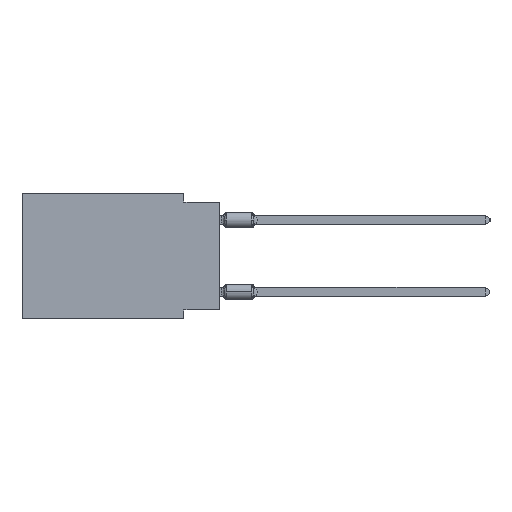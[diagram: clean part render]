
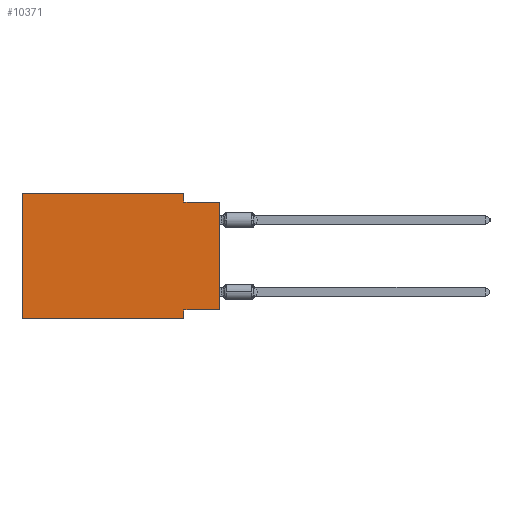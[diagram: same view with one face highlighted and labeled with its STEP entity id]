
A CAD part, left-side view. The second image highlights one B-rep face of the part: STEP entity #10371.
In plain terms, the highlighted planar face has unit normal (-1, 0, 0).
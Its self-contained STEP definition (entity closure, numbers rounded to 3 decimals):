
#61 = LINE ( 'NONE', #2309, #18541 ) ;
#2309 = CARTESIAN_POINT ( 'NONE',  ( 0., 13.97, 0. ) ) ;
#2545 = CARTESIAN_POINT ( 'NONE',  ( 0., 0., -8.255 ) ) ;
#3262 = CARTESIAN_POINT ( 'NONE',  ( 0., 13.97, 0. ) ) ;
#3660 = EDGE_CURVE ( 'NONE', #30574, #4912, #35117, .T. ) ;
#3674 = ORIENTED_EDGE ( 'NONE', *, *, #30436, .T. ) ;
#4912 = VERTEX_POINT ( 'NONE', #15477 ) ;
#5928 = ORIENTED_EDGE ( 'NONE', *, *, #24770, .F. ) ;
#6356 = VECTOR ( 'NONE', #14920, 1000. ) ;
#6431 = LINE ( 'NONE', #3262, #14366 ) ;
#7239 = DIRECTION ( 'NONE',  ( 1., 0., 0. ) ) ;
#7832 = VERTEX_POINT ( 'NONE', #29758 ) ;
#8662 = ORIENTED_EDGE ( 'NONE', *, *, #3660, .T. ) ;
#8764 = EDGE_CURVE ( 'NONE', #19651, #4912, #22939, .T. ) ;
#9481 = FACE_OUTER_BOUND ( 'NONE', #26219, .T. ) ;
#9772 = VERTEX_POINT ( 'NONE', #2545 ) ;
#10213 = ORIENTED_EDGE ( 'NONE', *, *, #8764, .F. ) ;
#10260 = LINE ( 'NONE', #21566, #25168 ) ;
#10371 = ADVANCED_FACE ( 'NONE', ( #9481 ), #20780, .F. ) ;
#12617 = CARTESIAN_POINT ( 'NONE',  ( 0., 13.97, 0. ) ) ;
#12958 = ORIENTED_EDGE ( 'NONE', *, *, #13366, .F. ) ;
#13186 = CARTESIAN_POINT ( 'NONE',  ( 0., 13.97, -8.89 ) ) ;
#13366 = EDGE_CURVE ( 'NONE', #30574, #7832, #6431, .T. ) ;
#13613 = CARTESIAN_POINT ( 'NONE',  ( 0., 0., -0.635 ) ) ;
#13700 = CARTESIAN_POINT ( 'NONE',  ( 0., 2.54, 0. ) ) ;
#14366 = VECTOR ( 'NONE', #14581, 1000. ) ;
#14581 = DIRECTION ( 'NONE',  ( 0., 0., 1. ) ) ;
#14920 = DIRECTION ( 'NONE',  ( 0., -1., 0. ) ) ;
#15048 = CARTESIAN_POINT ( 'NONE',  ( 0., 0., 0. ) ) ;
#15477 = CARTESIAN_POINT ( 'NONE',  ( 0., 2.54, -8.89 ) ) ;
#15602 = EDGE_CURVE ( 'NONE', #7832, #22359, #61, .T. ) ;
#16563 = LINE ( 'NONE', #15048, #26365 ) ;
#18491 = LINE ( 'NONE', #27394, #21129 ) ;
#18541 = VECTOR ( 'NONE', #33624, 1000. ) ;
#19112 = AXIS2_PLACEMENT_3D ( 'NONE', #12617, #7239, #23933 ) ;
#19426 = CARTESIAN_POINT ( 'NONE',  ( 0., 2.54, -8.89 ) ) ;
#19651 = VERTEX_POINT ( 'NONE', #22724 ) ;
#20051 = VERTEX_POINT ( 'NONE', #13613 ) ;
#20566 = ORIENTED_EDGE ( 'NONE', *, *, #23843, .F. ) ;
#20780 = PLANE ( 'NONE',  #19112 ) ;
#21129 = VECTOR ( 'NONE', #29786, 1000. ) ;
#21566 = CARTESIAN_POINT ( 'NONE',  ( 0., 0., -8.255 ) ) ;
#22359 = VERTEX_POINT ( 'NONE', #13700 ) ;
#22724 = CARTESIAN_POINT ( 'NONE',  ( 0., 2.54, -8.255 ) ) ;
#22939 = LINE ( 'NONE', #19426, #29709 ) ;
#23604 = DIRECTION ( 'NONE',  ( 0., 0., -1. ) ) ;
#23843 = EDGE_CURVE ( 'NONE', #35927, #20051, #18491, .T. ) ;
#23933 = DIRECTION ( 'NONE',  ( 0., 0., -1. ) ) ;
#24770 = EDGE_CURVE ( 'NONE', #22359, #35927, #35263, .T. ) ;
#25168 = VECTOR ( 'NONE', #30088, 1000. ) ;
#26219 = EDGE_LOOP ( 'NONE', ( #3674, #20566, #5928, #31090, #12958, #8662, #10213, #33894 ) ) ;
#26365 = VECTOR ( 'NONE', #35067, 1000. ) ;
#26941 = CARTESIAN_POINT ( 'NONE',  ( 0., 2.54, 0. ) ) ;
#27394 = CARTESIAN_POINT ( 'NONE',  ( 0., 0., -0.635 ) ) ;
#29709 = VECTOR ( 'NONE', #34228, 1000. ) ;
#29758 = CARTESIAN_POINT ( 'NONE',  ( 0., 13.97, 0. ) ) ;
#29786 = DIRECTION ( 'NONE',  ( 0., -1., 0. ) ) ;
#30088 = DIRECTION ( 'NONE',  ( 0., 1., 0. ) ) ;
#30296 = EDGE_CURVE ( 'NONE', #9772, #19651, #10260, .T. ) ;
#30436 = EDGE_CURVE ( 'NONE', #9772, #20051, #16563, .T. ) ;
#30574 = VERTEX_POINT ( 'NONE', #13186 ) ;
#31090 = ORIENTED_EDGE ( 'NONE', *, *, #15602, .F. ) ;
#31978 = CARTESIAN_POINT ( 'NONE',  ( 0., 13.97, -8.89 ) ) ;
#33624 = DIRECTION ( 'NONE',  ( 0., -1., 0. ) ) ;
#33894 = ORIENTED_EDGE ( 'NONE', *, *, #30296, .F. ) ;
#34121 = CARTESIAN_POINT ( 'NONE',  ( 0., 2.54, -0.635 ) ) ;
#34228 = DIRECTION ( 'NONE',  ( 0., 0., -1. ) ) ;
#35067 = DIRECTION ( 'NONE',  ( 0., 0., 1. ) ) ;
#35117 = LINE ( 'NONE', #31978, #6356 ) ;
#35263 = LINE ( 'NONE', #26941, #35359 ) ;
#35359 = VECTOR ( 'NONE', #23604, 1000. ) ;
#35927 = VERTEX_POINT ( 'NONE', #34121 ) ;
